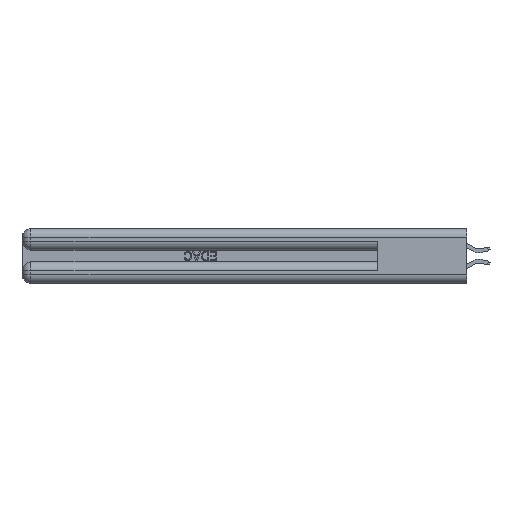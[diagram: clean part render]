
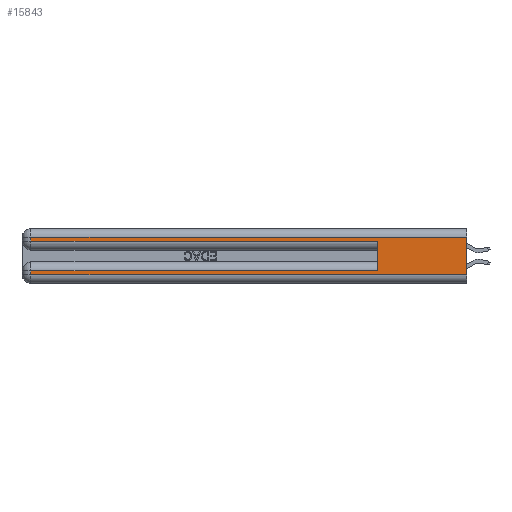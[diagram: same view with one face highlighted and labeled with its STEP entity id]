
A CAD part, left-side view. The second image highlights one B-rep face of the part: STEP entity #15843.
In plain terms, the highlighted planar face has unit normal (-1, 0, 0).
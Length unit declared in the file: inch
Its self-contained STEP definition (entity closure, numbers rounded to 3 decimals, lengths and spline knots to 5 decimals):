
#250 = CARTESIAN_POINT ( 'NONE',  ( 0., 0., 0.31 ) ) ;
#315 = CARTESIAN_POINT ( 'NONE',  ( 0., 0., 0.085 ) ) ;
#967 = CARTESIAN_POINT ( 'NONE',  ( 0., 2.94, 0.37 ) ) ;
#1193 = EDGE_CURVE ( 'NONE', #20547, #23741, #12772, .T. ) ;
#2552 = DIRECTION ( 'NONE',  ( 0., 0., -1. ) ) ;
#2679 = EDGE_CURVE ( 'NONE', #30294, #32150, #37358, .T. ) ;
#3864 = VERTEX_POINT ( 'NONE', #250 ) ;
#5325 = EDGE_CURVE ( 'NONE', #20547, #30294, #33849, .T. ) ;
#5362 = CARTESIAN_POINT ( 'NONE',  ( 0., 2.94, 0.285 ) ) ;
#6670 = CARTESIAN_POINT ( 'NONE',  ( 0., 0.6, 0.145 ) ) ;
#6760 = DIRECTION ( 'NONE',  ( 1., 0., 0. ) ) ;
#7748 = VERTEX_POINT ( 'NONE', #5362 ) ;
#9511 = CARTESIAN_POINT ( 'NONE',  ( 0., 2.94, 0.06 ) ) ;
#10618 = EDGE_CURVE ( 'NONE', #32150, #42409, #26222, .T. ) ;
#11525 = DIRECTION ( 'NONE',  ( 0., -1., 0. ) ) ;
#11586 = DIRECTION ( 'NONE',  ( 0., 0., -1. ) ) ;
#11610 = DIRECTION ( 'NONE',  ( 0., 0., -1. ) ) ;
#11865 = VECTOR ( 'NONE', #11586, 39.37008 ) ;
#11886 = ORIENTED_EDGE ( 'NONE', *, *, #36805, .T. ) ;
#12772 = LINE ( 'NONE', #6670, #14981 ) ;
#12870 = EDGE_LOOP ( 'NONE', ( #44254, #22921, #17388, #11886, #23461, #15212, #39366, #15788 ) ) ;
#14981 = VECTOR ( 'NONE', #31209, 39.37008 ) ;
#15212 = ORIENTED_EDGE ( 'NONE', *, *, #5325, .T. ) ;
#15788 = ORIENTED_EDGE ( 'NONE', *, *, #10618, .T. ) ;
#15843 = ADVANCED_FACE ( 'NONE', ( #22102 ), #17251, .F. ) ;
#17151 = VECTOR ( 'NONE', #28270, 39.37008 ) ;
#17251 = PLANE ( 'NONE',  #45050 ) ;
#17388 = ORIENTED_EDGE ( 'NONE', *, *, #34668, .T. ) ;
#18057 = DIRECTION ( 'NONE',  ( 0., 1., 0. ) ) ;
#18827 = VECTOR ( 'NONE', #2552, 39.37008 ) ;
#19928 = LINE ( 'NONE', #20140, #18827 ) ;
#20140 = CARTESIAN_POINT ( 'NONE',  ( 0., 0., 0.37 ) ) ;
#20547 = VERTEX_POINT ( 'NONE', #39022 ) ;
#22102 = FACE_OUTER_BOUND ( 'NONE', #12870, .T. ) ;
#22921 = ORIENTED_EDGE ( 'NONE', *, *, #42645, .T. ) ;
#23436 = CARTESIAN_POINT ( 'NONE',  ( 0., 0., 0.285 ) ) ;
#23461 = ORIENTED_EDGE ( 'NONE', *, *, #1193, .F. ) ;
#23741 = VERTEX_POINT ( 'NONE', #40369 ) ;
#24202 = CARTESIAN_POINT ( 'NONE',  ( 0., 0., 0.06 ) ) ;
#24538 = VECTOR ( 'NONE', #18057, 39.37008 ) ;
#25525 = EDGE_CURVE ( 'NONE', #3864, #42409, #19928, .T. ) ;
#26222 = LINE ( 'NONE', #39626, #35577 ) ;
#27954 = CARTESIAN_POINT ( 'NONE',  ( 0., 2.94, 0.31 ) ) ;
#27969 = VECTOR ( 'NONE', #11610, 39.37008 ) ;
#28270 = DIRECTION ( 'NONE',  ( 0., 1., 0. ) ) ;
#29061 = CARTESIAN_POINT ( 'NONE',  ( 0., 2.94, 0.37 ) ) ;
#30294 = VERTEX_POINT ( 'NONE', #38349 ) ;
#31209 = DIRECTION ( 'NONE',  ( 0., 0., 1. ) ) ;
#31299 = DIRECTION ( 'NONE',  ( 0., 0., -1. ) ) ;
#32150 = VERTEX_POINT ( 'NONE', #9511 ) ;
#32709 = LINE ( 'NONE', #967, #11865 ) ;
#33007 = VERTEX_POINT ( 'NONE', #27954 ) ;
#33849 = LINE ( 'NONE', #315, #24538 ) ;
#34668 = EDGE_CURVE ( 'NONE', #33007, #7748, #32709, .T. ) ;
#35235 = VECTOR ( 'NONE', #41052, 39.37008 ) ;
#35353 = CARTESIAN_POINT ( 'NONE',  ( 0., 0., 0.31 ) ) ;
#35577 = VECTOR ( 'NONE', #11525, 39.37008 ) ;
#36805 = EDGE_CURVE ( 'NONE', #7748, #23741, #44631, .T. ) ;
#36903 = LINE ( 'NONE', #35353, #17151 ) ;
#37358 = LINE ( 'NONE', #29061, #27969 ) ;
#38349 = CARTESIAN_POINT ( 'NONE',  ( 0., 2.94, 0.085 ) ) ;
#39022 = CARTESIAN_POINT ( 'NONE',  ( 0., 0.6, 0.085 ) ) ;
#39366 = ORIENTED_EDGE ( 'NONE', *, *, #2679, .T. ) ;
#39626 = CARTESIAN_POINT ( 'NONE',  ( 0., 0., 0.06 ) ) ;
#40369 = CARTESIAN_POINT ( 'NONE',  ( 0., 0.6, 0.285 ) ) ;
#41052 = DIRECTION ( 'NONE',  ( 0., -1., 0. ) ) ;
#42409 = VERTEX_POINT ( 'NONE', #24202 ) ;
#42645 = EDGE_CURVE ( 'NONE', #3864, #33007, #36903, .T. ) ;
#44254 = ORIENTED_EDGE ( 'NONE', *, *, #25525, .F. ) ;
#44631 = LINE ( 'NONE', #23436, #35235 ) ;
#45050 = AXIS2_PLACEMENT_3D ( 'NONE', #45306, #6760, #31299 ) ;
#45306 = CARTESIAN_POINT ( 'NONE',  ( 0., 0., 0.37 ) ) ;
